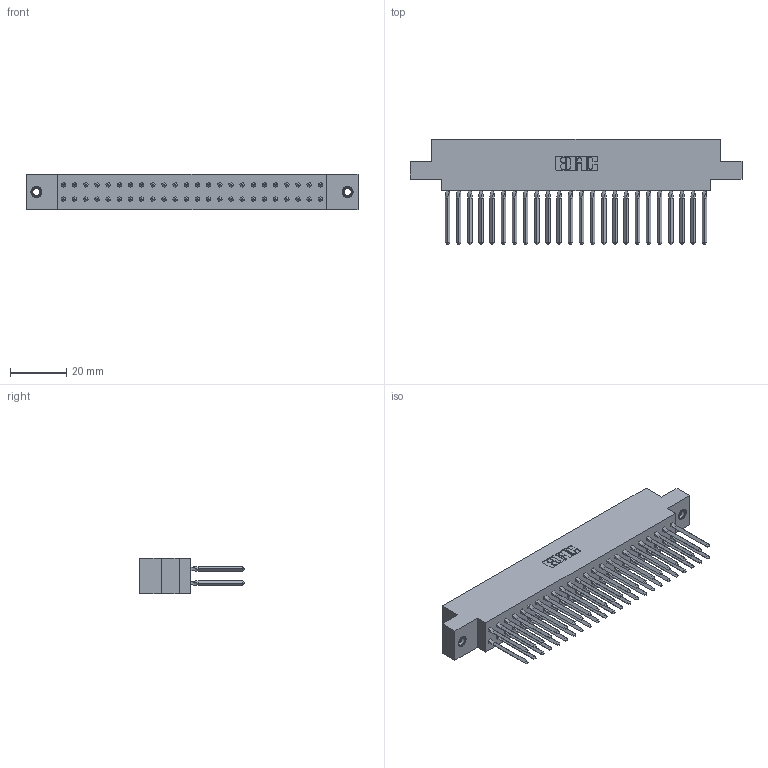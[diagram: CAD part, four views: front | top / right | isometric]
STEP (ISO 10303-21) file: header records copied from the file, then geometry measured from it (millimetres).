
FILE_DESCRIPTION (( 'STEP AP203' ), '1' );
FILE_NAME ('317-048-542-807.STEP', '2020-02-28T02:51:04', ( '' ), ( '' ), 'SwSTEP 2.0', 'SolidWorks 2016', '' );
FILE_SCHEMA (( 'CONFIG_CONTROL_DESIGN' ));
Length unit declared in the file: inch
Products named in the file (4): 317-048-542-807; 317-290-003_542; 345-250-001_345-250-005-103; 317 Part_.156 Dia - TI
Assembly tree (51 placements, depth 2):
  317-048-542-807
    317 Part_.156 Dia - TI
    317-290-003_542  x48
    345-250-001_345-250-005-103  x2
Bounding box: 117.81 x 37.34 x 12.7 mm (x, y, z)
Volume: 18707.8 mm3; surface area: 25473.8 mm2
Topology: 51 solids, 51 shells, 2898 faces, 8091 edges, 5162 vertices
Faces by surface type: plane 2298, cylinder 392, bspline 192, cone 12, torus 4
Entity records: 37406 total; most frequent: CARTESIAN_POINT 6744, ORIENTED_EDGE 6400, DIRECTION 5454, EDGE_CURVE 3200, LINE 3010, VECTOR 3010, VERTEX_POINT 2124, AXIS2_PLACEMENT_3D 1222
